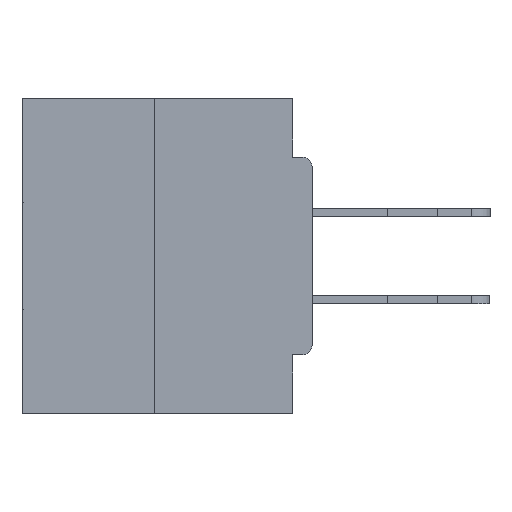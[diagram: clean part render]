
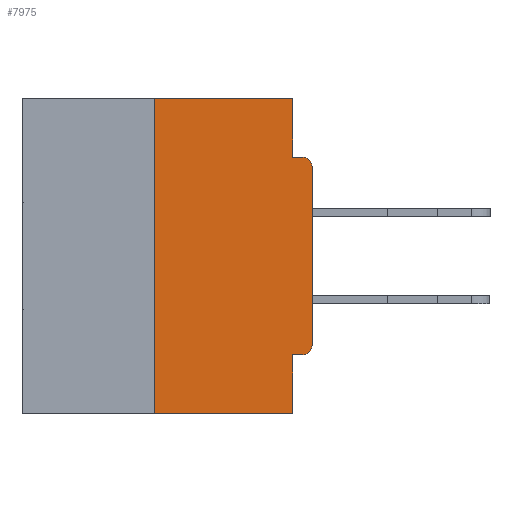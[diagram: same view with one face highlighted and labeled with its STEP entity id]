
A CAD part, left-side view. The second image highlights one B-rep face of the part: STEP entity #7975.
In plain terms, the highlighted planar face has unit normal (-1, 0, 0).
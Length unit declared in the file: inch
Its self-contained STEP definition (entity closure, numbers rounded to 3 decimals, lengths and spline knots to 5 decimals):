
#337 = CARTESIAN_POINT ( 'NONE',  ( 0., 0.015, -0.1085 ) ) ;
#1966 = VERTEX_POINT ( 'NONE', #38575 ) ;
#2167 = DIRECTION ( 'NONE',  ( 1., 0., 0. ) ) ;
#2187 = EDGE_CURVE ( 'NONE', #2372, #18712, #18842, .T. ) ;
#2372 = VERTEX_POINT ( 'NONE', #30962 ) ;
#3126 = EDGE_CURVE ( 'NONE', #9724, #3355, #37651, .T. ) ;
#3298 = LINE ( 'NONE', #27941, #22685 ) ;
#3355 = VERTEX_POINT ( 'NONE', #12608 ) ;
#4075 = DIRECTION ( 'NONE',  ( 0., 0., 1. ) ) ;
#4672 = AXIS2_PLACEMENT_3D ( 'NONE', #337, #9553, #18372 ) ;
#4707 = LINE ( 'NONE', #26319, #40061 ) ;
#5330 = EDGE_CURVE ( 'NONE', #5443, #3355, #4707, .T. ) ;
#5443 = VERTEX_POINT ( 'NONE', #8654 ) ;
#7470 = EDGE_CURVE ( 'NONE', #32823, #2372, #38941, .T. ) ;
#7975 = ADVANCED_FACE ( 'NONE', ( #9344 ), #26743, .F. ) ;
#8614 = EDGE_CURVE ( 'NONE', #32019, #18712, #22373, .T. ) ;
#8654 = CARTESIAN_POINT ( 'NONE',  ( 0., 0.031, -0.4065 ) ) ;
#9090 = DIRECTION ( 'NONE',  ( 0., 0., -1. ) ) ;
#9344 = FACE_OUTER_BOUND ( 'NONE', #32683, .T. ) ;
#9553 = DIRECTION ( 'NONE',  ( -1., 0., 0. ) ) ;
#9724 = VERTEX_POINT ( 'NONE', #23359 ) ;
#9728 = CARTESIAN_POINT ( 'NONE',  ( 0., 0., 0. ) ) ;
#10369 = CIRCLE ( 'NONE', #13360, 0.015 ) ;
#10744 = VECTOR ( 'NONE', #14770, 39.37008 ) ;
#12392 = AXIS2_PLACEMENT_3D ( 'NONE', #36038, #2167, #17777 ) ;
#12463 = EDGE_CURVE ( 'NONE', #1966, #5443, #26487, .T. ) ;
#12608 = CARTESIAN_POINT ( 'NONE',  ( 0., 0.031, -0.5 ) ) ;
#13016 = ORIENTED_EDGE ( 'NONE', *, *, #3126, .T. ) ;
#13360 = AXIS2_PLACEMENT_3D ( 'NONE', #24029, #39294, #9090 ) ;
#14401 = EDGE_CURVE ( 'NONE', #28898, #32823, #18987, .T. ) ;
#14770 = DIRECTION ( 'NONE',  ( 0., -1., 0. ) ) ;
#15130 = DIRECTION ( 'NONE',  ( 0., -1., 0. ) ) ;
#15575 = LINE ( 'NONE', #9728, #25335 ) ;
#17730 = DIRECTION ( 'NONE',  ( 0., 1., 0. ) ) ;
#17777 = DIRECTION ( 'NONE',  ( 0., 0., -1. ) ) ;
#18372 = DIRECTION ( 'NONE',  ( 0., 0., -1. ) ) ;
#18549 = DIRECTION ( 'NONE',  ( 0., 0., 1. ) ) ;
#18712 = VERTEX_POINT ( 'NONE', #23750 ) ;
#18842 = LINE ( 'NONE', #27673, #22751 ) ;
#18987 = LINE ( 'NONE', #23495, #10744 ) ;
#19040 = ORIENTED_EDGE ( 'NONE', *, *, #12463, .F. ) ;
#20561 = CARTESIAN_POINT ( 'NONE',  ( 0., 0., -0.4065 ) ) ;
#21798 = ORIENTED_EDGE ( 'NONE', *, *, #2187, .F. ) ;
#22098 = ORIENTED_EDGE ( 'NONE', *, *, #34684, .T. ) ;
#22373 = CIRCLE ( 'NONE', #4672, 0.015 ) ;
#22685 = VECTOR ( 'NONE', #4075, 39.37008 ) ;
#22751 = VECTOR ( 'NONE', #15130, 39.37008 ) ;
#22948 = ORIENTED_EDGE ( 'NONE', *, *, #5330, .F. ) ;
#23178 = DIRECTION ( 'NONE',  ( 0., 0., -1. ) ) ;
#23359 = CARTESIAN_POINT ( 'NONE',  ( 0., 0.25, -0.5 ) ) ;
#23495 = CARTESIAN_POINT ( 'NONE',  ( 0., 0.46, 0. ) ) ;
#23511 = CARTESIAN_POINT ( 'NONE',  ( 0., 0.25, 0. ) ) ;
#23619 = VECTOR ( 'NONE', #27029, 39.37008 ) ;
#23750 = CARTESIAN_POINT ( 'NONE',  ( 0., 0.015, -0.0935 ) ) ;
#24029 = CARTESIAN_POINT ( 'NONE',  ( 0., 0.015, -0.3915 ) ) ;
#25335 = VECTOR ( 'NONE', #18549, 39.37008 ) ;
#26319 = CARTESIAN_POINT ( 'NONE',  ( 0., 0.031, -0.5 ) ) ;
#26487 = LINE ( 'NONE', #20561, #35137 ) ;
#26743 = PLANE ( 'NONE',  #12392 ) ;
#27029 = DIRECTION ( 'NONE',  ( 0., -1., 0. ) ) ;
#27673 = CARTESIAN_POINT ( 'NONE',  ( 0., 0., -0.0935 ) ) ;
#27941 = CARTESIAN_POINT ( 'NONE',  ( 0., 0.25, 0. ) ) ;
#28898 = VERTEX_POINT ( 'NONE', #23511 ) ;
#30768 = VECTOR ( 'NONE', #23178, 39.37008 ) ;
#30832 = CARTESIAN_POINT ( 'NONE',  ( 0., 0.031, 0. ) ) ;
#30962 = CARTESIAN_POINT ( 'NONE',  ( 0., 0.031, -0.0935 ) ) ;
#31344 = ORIENTED_EDGE ( 'NONE', *, *, #14401, .F. ) ;
#31724 = EDGE_CURVE ( 'NONE', #9724, #28898, #3298, .T. ) ;
#32019 = VERTEX_POINT ( 'NONE', #33274 ) ;
#32683 = EDGE_LOOP ( 'NONE', ( #31344, #37509, #13016, #22948, #19040, #34282, #22098, #37675, #21798, #32782 ) ) ;
#32782 = ORIENTED_EDGE ( 'NONE', *, *, #7470, .F. ) ;
#32823 = VERTEX_POINT ( 'NONE', #30832 ) ;
#33274 = CARTESIAN_POINT ( 'NONE',  ( 0., 0., -0.1085 ) ) ;
#34282 = ORIENTED_EDGE ( 'NONE', *, *, #39613, .T. ) ;
#34684 = EDGE_CURVE ( 'NONE', #39399, #32019, #15575, .T. ) ;
#35137 = VECTOR ( 'NONE', #17730, 39.37008 ) ;
#35336 = CARTESIAN_POINT ( 'NONE',  ( 0., 0.031, 0. ) ) ;
#36038 = CARTESIAN_POINT ( 'NONE',  ( 0., 0.46, 0. ) ) ;
#37509 = ORIENTED_EDGE ( 'NONE', *, *, #31724, .F. ) ;
#37651 = LINE ( 'NONE', #39305, #23619 ) ;
#37675 = ORIENTED_EDGE ( 'NONE', *, *, #8614, .T. ) ;
#37830 = CARTESIAN_POINT ( 'NONE',  ( 0., 0., -0.3915 ) ) ;
#38575 = CARTESIAN_POINT ( 'NONE',  ( 0., 0.015, -0.4065 ) ) ;
#38729 = DIRECTION ( 'NONE',  ( 0., 0., -1. ) ) ;
#38941 = LINE ( 'NONE', #35336, #30768 ) ;
#39294 = DIRECTION ( 'NONE',  ( -1., 0., 0. ) ) ;
#39305 = CARTESIAN_POINT ( 'NONE',  ( 0., 0.46, -0.5 ) ) ;
#39399 = VERTEX_POINT ( 'NONE', #37830 ) ;
#39613 = EDGE_CURVE ( 'NONE', #1966, #39399, #10369, .T. ) ;
#40061 = VECTOR ( 'NONE', #38729, 39.37008 ) ;
